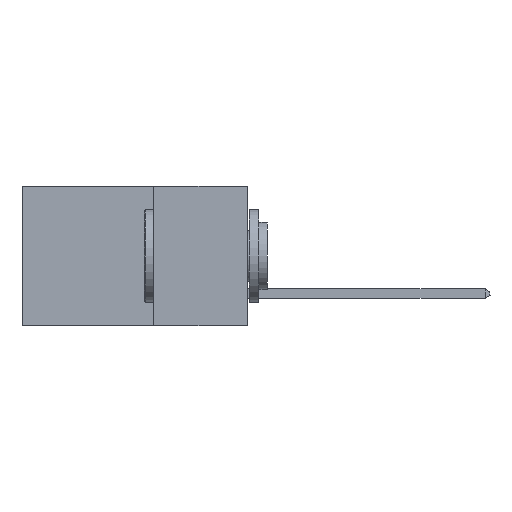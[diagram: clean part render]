
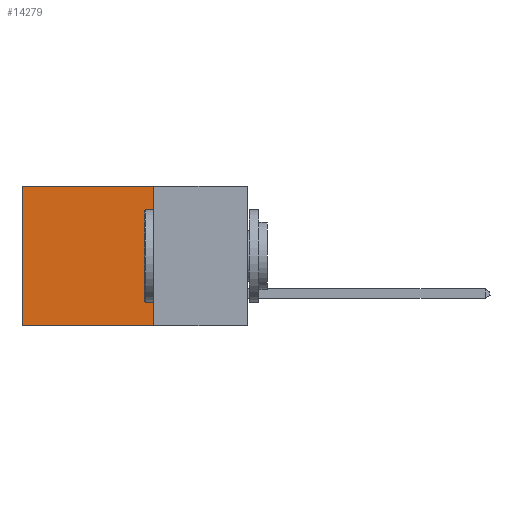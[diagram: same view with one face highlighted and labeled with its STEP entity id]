
A CAD part, left-side view. The second image highlights one B-rep face of the part: STEP entity #14279.
In plain terms, the highlighted planar face has unit normal (-1, 0, 0).
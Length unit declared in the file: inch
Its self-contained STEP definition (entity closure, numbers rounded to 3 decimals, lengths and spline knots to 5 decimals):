
#106 = DIRECTION ( 'NONE',  ( 1., 0., 0. ) ) ;
#411 = DIRECTION ( 'NONE',  ( 0., 0., -1. ) ) ;
#615 = LINE ( 'NONE', #8924, #12014 ) ;
#1169 = FACE_OUTER_BOUND ( 'NONE', #12409, .T. ) ;
#2607 = AXIS2_PLACEMENT_3D ( 'NONE', #11474, #106, #18326 ) ;
#3231 = PLANE ( 'NONE',  #2607 ) ;
#3720 = CARTESIAN_POINT ( 'NONE',  ( 0.298, 0.25, 0. ) ) ;
#3945 = CARTESIAN_POINT ( 'NONE',  ( 0.298, 0.25, -0.37 ) ) ;
#4182 = VECTOR ( 'NONE', #8868, 39.37008 ) ;
#4632 = LINE ( 'NONE', #5540, #9041 ) ;
#5540 = CARTESIAN_POINT ( 'NONE',  ( 0.298, 0.6, 0. ) ) ;
#6038 = LINE ( 'NONE', #3945, #11998 ) ;
#6566 = CARTESIAN_POINT ( 'NONE',  ( 0.298, 0.25, -0.37 ) ) ;
#7236 = CARTESIAN_POINT ( 'NONE',  ( 0.298, 0.25, 0. ) ) ;
#7736 = VERTEX_POINT ( 'NONE', #6566 ) ;
#8592 = LINE ( 'NONE', #3720, #4182 ) ;
#8868 = DIRECTION ( 'NONE',  ( 0., 0., -1. ) ) ;
#8924 = CARTESIAN_POINT ( 'NONE',  ( 0.298, 0.25, 0. ) ) ;
#9041 = VECTOR ( 'NONE', #411, 39.37008 ) ;
#9560 = EDGE_CURVE ( 'NONE', #15217, #17202, #4632, .T. ) ;
#11474 = CARTESIAN_POINT ( 'NONE',  ( 0.298, 0.25, 0. ) ) ;
#11998 = VECTOR ( 'NONE', #18858, 39.37008 ) ;
#12014 = VECTOR ( 'NONE', #12042, 39.37008 ) ;
#12042 = DIRECTION ( 'NONE',  ( 0., 1., 0. ) ) ;
#12343 = ORIENTED_EDGE ( 'NONE', *, *, #14911, .F. ) ;
#12409 = EDGE_LOOP ( 'NONE', ( #15757, #12343, #18553, #13646 ) ) ;
#13231 = CARTESIAN_POINT ( 'NONE',  ( 0.298, 0.6, -0.37 ) ) ;
#13646 = ORIENTED_EDGE ( 'NONE', *, *, #21045, .T. ) ;
#14079 = VERTEX_POINT ( 'NONE', #7236 ) ;
#14279 = ADVANCED_FACE ( 'NONE', ( #1169 ), #3231, .F. ) ;
#14911 = EDGE_CURVE ( 'NONE', #7736, #17202, #6038, .T. ) ;
#15217 = VERTEX_POINT ( 'NONE', #18303 ) ;
#15757 = ORIENTED_EDGE ( 'NONE', *, *, #9560, .T. ) ;
#15997 = EDGE_CURVE ( 'NONE', #14079, #7736, #8592, .T. ) ;
#17202 = VERTEX_POINT ( 'NONE', #13231 ) ;
#18303 = CARTESIAN_POINT ( 'NONE',  ( 0.298, 0.6, 0. ) ) ;
#18326 = DIRECTION ( 'NONE',  ( 0., 0., -1. ) ) ;
#18553 = ORIENTED_EDGE ( 'NONE', *, *, #15997, .F. ) ;
#18858 = DIRECTION ( 'NONE',  ( 0., 1., 0. ) ) ;
#21045 = EDGE_CURVE ( 'NONE', #14079, #15217, #615, .T. ) ;
